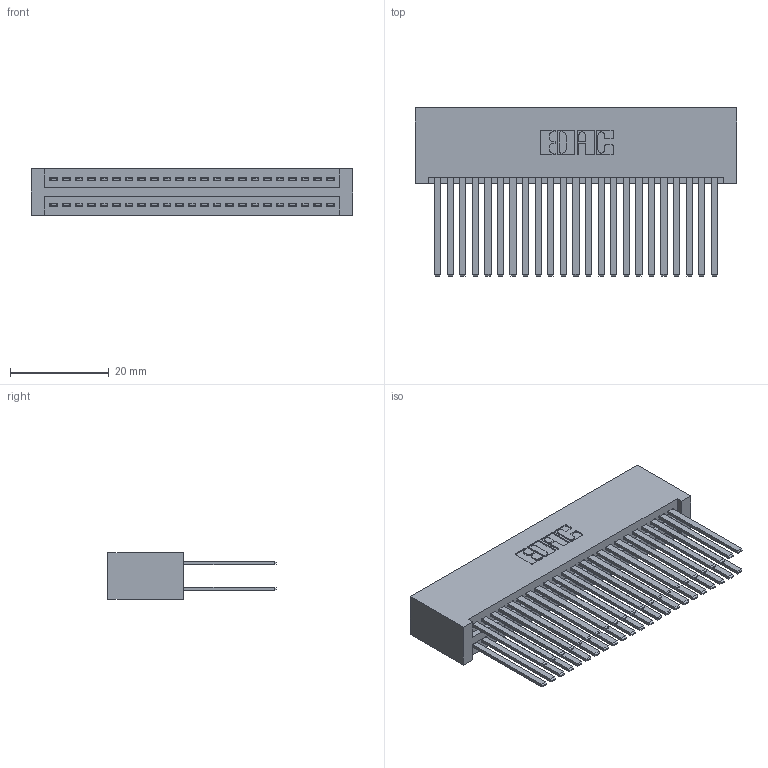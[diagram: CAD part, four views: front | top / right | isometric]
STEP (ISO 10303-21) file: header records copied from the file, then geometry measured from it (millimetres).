
FILE_DESCRIPTION (( 'STEP AP203' ), '1' );
FILE_NAME ('395-046-544-201.STEP', '2019-10-19T04:13:54', ( '' ), ( '' ), 'SwSTEP 2.0', 'SolidWorks 2016', '' );
FILE_SCHEMA (( 'CONFIG_CONTROL_DESIGN' ));
Length unit declared in the file: inch
Products named in the file (3): 345 Part_No Mounting Lugs; 345-292-001_345-293-144; 395-046-544-201
Assembly tree (47 placements, depth 2):
  395-046-544-201
    345 Part_No Mounting Lugs
    345-292-001_345-293-144  x46
Bounding box: 65.02 x 33.96 x 9.4 mm (x, y, z)
Volume: 7400.9 mm3; surface area: 12765 mm2
Topology: 47 solids, 47 shells, 2142 faces, 6343 edges, 4166 vertices
Faces by surface type: plane 1410, cylinder 732
Entity records: 20143 total; most frequent: CARTESIAN_POINT 3392, ORIENTED_EDGE 3326, DIRECTION 3007, EDGE_CURVE 1663, LINE 1451, VECTOR 1451, VERTEX_POINT 1106, AXIS2_PLACEMENT_3D 778
